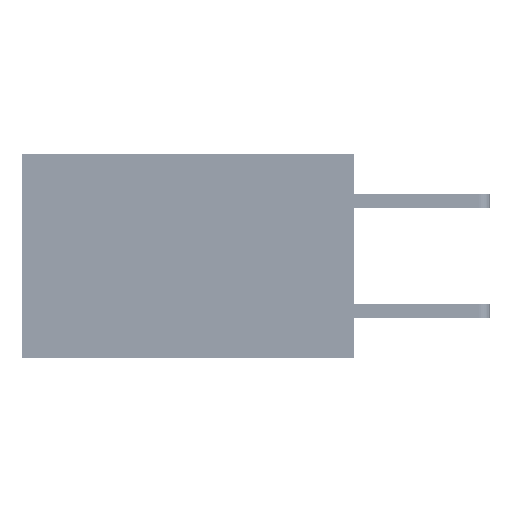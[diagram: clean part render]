
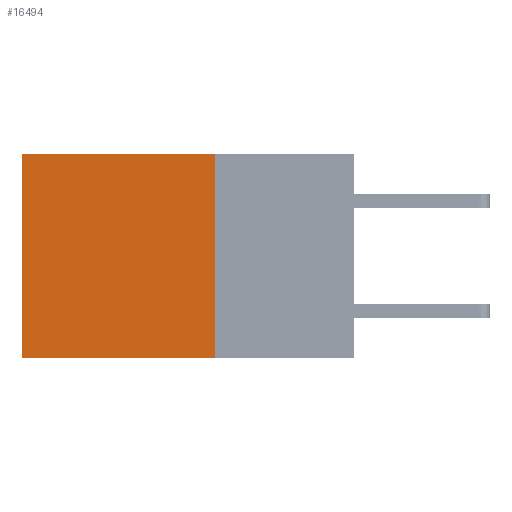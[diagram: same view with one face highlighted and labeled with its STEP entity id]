
A CAD part, left-side view. The second image highlights one B-rep face of the part: STEP entity #16494.
In plain terms, the highlighted planar face has unit normal (-1, 0, 0).
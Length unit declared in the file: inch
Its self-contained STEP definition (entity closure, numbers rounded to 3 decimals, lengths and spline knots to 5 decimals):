
#3005 = ORIENTED_EDGE ( 'NONE', *, *, #4366, .T. ) ;
#4366 = EDGE_CURVE ( 'NONE', #18103, #12536, #16972, .T. ) ;
#11211 = DIRECTION ( 'NONE',  ( 0., 0., -1. ) ) ;
#11676 = CARTESIAN_POINT ( 'NONE',  ( 0.2875, 0.25, 0. ) ) ;
#11979 = CARTESIAN_POINT ( 'NONE',  ( 0.2875, 0.25, 0. ) ) ;
#12536 = VERTEX_POINT ( 'NONE', #39443 ) ;
#13619 = CARTESIAN_POINT ( 'NONE',  ( 0.2875, 0.25, -0.37 ) ) ;
#15189 = VECTOR ( 'NONE', #49860, 39.37008 ) ;
#15402 = EDGE_CURVE ( 'NONE', #49134, #12536, #46377, .T. ) ;
#16148 = VERTEX_POINT ( 'NONE', #11676 ) ;
#16494 = ADVANCED_FACE ( 'NONE', ( #16868 ), #22293, .F. ) ;
#16831 = LINE ( 'NONE', #11979, #49900 ) ;
#16868 = FACE_OUTER_BOUND ( 'NONE', #19360, .T. ) ;
#16972 = LINE ( 'NONE', #23504, #48767 ) ;
#17771 = LINE ( 'NONE', #33202, #15189 ) ;
#18103 = VERTEX_POINT ( 'NONE', #52694 ) ;
#19222 = ORIENTED_EDGE ( 'NONE', *, *, #43152, .F. ) ;
#19360 = EDGE_LOOP ( 'NONE', ( #3005, #46510, #19222, #43479 ) ) ;
#22293 = PLANE ( 'NONE',  #50423 ) ;
#23504 = CARTESIAN_POINT ( 'NONE',  ( 0.2875, 0.6, 0. ) ) ;
#27900 = DIRECTION ( 'NONE',  ( 0., 0., -1. ) ) ;
#29376 = EDGE_CURVE ( 'NONE', #16148, #18103, #17771, .T. ) ;
#31063 = CARTESIAN_POINT ( 'NONE',  ( 0.2875, 0.25, -0.37 ) ) ;
#33202 = CARTESIAN_POINT ( 'NONE',  ( 0.2875, 0.25, 0. ) ) ;
#38452 = DIRECTION ( 'NONE',  ( 1., 0., 0. ) ) ;
#38624 = CARTESIAN_POINT ( 'NONE',  ( 0.2875, 0.25, 0. ) ) ;
#39443 = CARTESIAN_POINT ( 'NONE',  ( 0.2875, 0.6, -0.37 ) ) ;
#43139 = VECTOR ( 'NONE', #47217, 39.37008 ) ;
#43152 = EDGE_CURVE ( 'NONE', #16148, #49134, #16831, .T. ) ;
#43479 = ORIENTED_EDGE ( 'NONE', *, *, #29376, .T. ) ;
#46377 = LINE ( 'NONE', #31063, #43139 ) ;
#46510 = ORIENTED_EDGE ( 'NONE', *, *, #15402, .F. ) ;
#47217 = DIRECTION ( 'NONE',  ( 0., 1., 0. ) ) ;
#48767 = VECTOR ( 'NONE', #11211, 39.37008 ) ;
#49134 = VERTEX_POINT ( 'NONE', #13619 ) ;
#49860 = DIRECTION ( 'NONE',  ( 0., 1., 0. ) ) ;
#49900 = VECTOR ( 'NONE', #27900, 39.37008 ) ;
#50423 = AXIS2_PLACEMENT_3D ( 'NONE', #38624, #38452, #51274 ) ;
#51274 = DIRECTION ( 'NONE',  ( 0., 0., -1. ) ) ;
#52694 = CARTESIAN_POINT ( 'NONE',  ( 0.2875, 0.6, 0. ) ) ;
